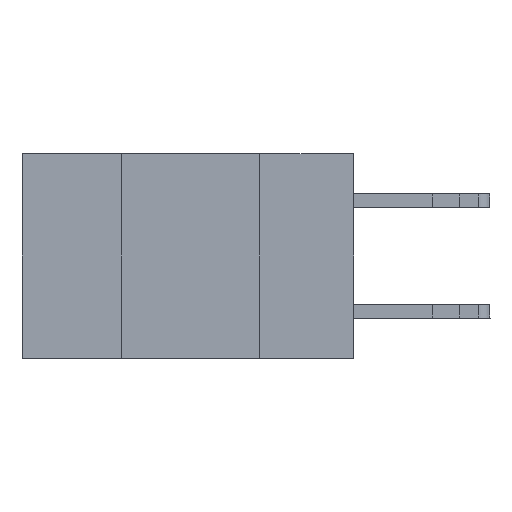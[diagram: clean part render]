
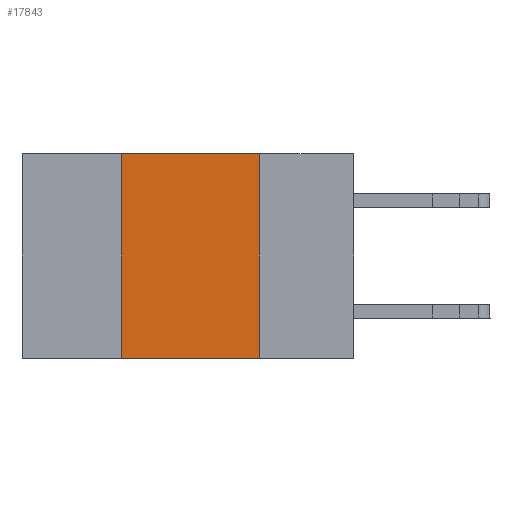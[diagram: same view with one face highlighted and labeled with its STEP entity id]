
A CAD part, left-side view. The second image highlights one B-rep face of the part: STEP entity #17843.
In plain terms, the highlighted planar face has unit normal (-1, 0, 0).
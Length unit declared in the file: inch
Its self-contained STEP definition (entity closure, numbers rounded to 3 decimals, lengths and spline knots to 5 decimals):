
#76 = CARTESIAN_POINT ( 'NONE',  ( 0., 0.6, 0. ) ) ;
#543 = ORIENTED_EDGE ( 'NONE', *, *, #3836, .F. ) ;
#1004 = LINE ( 'NONE', #16414, #1971 ) ;
#1146 = ORIENTED_EDGE ( 'NONE', *, *, #10322, .T. ) ;
#1477 = FACE_OUTER_BOUND ( 'NONE', #8916, .T. ) ;
#1574 = PLANE ( 'NONE',  #15258 ) ;
#1856 = CARTESIAN_POINT ( 'NONE',  ( 0., 0.42, 0. ) ) ;
#1971 = VECTOR ( 'NONE', #13468, 39.37008 ) ;
#2335 = CARTESIAN_POINT ( 'NONE',  ( 0., 0.42, -0.37 ) ) ;
#2457 = LINE ( 'NONE', #8667, #14725 ) ;
#3836 = EDGE_CURVE ( 'NONE', #6164, #16269, #12143, .T. ) ;
#4423 = DIRECTION ( 'NONE',  ( 1., 0., 0. ) ) ;
#5295 = CARTESIAN_POINT ( 'NONE',  ( 0., 0.17, -0.37 ) ) ;
#6164 = VERTEX_POINT ( 'NONE', #1856 ) ;
#7661 = LINE ( 'NONE', #13633, #12698 ) ;
#8169 = EDGE_CURVE ( 'NONE', #10997, #6164, #1004, .T. ) ;
#8365 = ORIENTED_EDGE ( 'NONE', *, *, #8169, .F. ) ;
#8667 = CARTESIAN_POINT ( 'NONE',  ( 0., 0.17, 0. ) ) ;
#8916 = EDGE_LOOP ( 'NONE', ( #16195, #543, #8365, #1146 ) ) ;
#10322 = EDGE_CURVE ( 'NONE', #10997, #15309, #7661, .T. ) ;
#10779 = DIRECTION ( 'NONE',  ( 0., 0., -1. ) ) ;
#10997 = VERTEX_POINT ( 'NONE', #2335 ) ;
#11593 = VECTOR ( 'NONE', #16829, 39.37008 ) ;
#12143 = LINE ( 'NONE', #18355, #11593 ) ;
#12698 = VECTOR ( 'NONE', #13937, 39.37008 ) ;
#12846 = CARTESIAN_POINT ( 'NONE',  ( 0., 0.17, 0. ) ) ;
#13468 = DIRECTION ( 'NONE',  ( 0., 0., 1. ) ) ;
#13633 = CARTESIAN_POINT ( 'NONE',  ( 0., 0.6, -0.37 ) ) ;
#13855 = DIRECTION ( 'NONE',  ( 0., 0., -1. ) ) ;
#13937 = DIRECTION ( 'NONE',  ( 0., -1., 0. ) ) ;
#14725 = VECTOR ( 'NONE', #10779, 39.37008 ) ;
#15258 = AXIS2_PLACEMENT_3D ( 'NONE', #76, #4423, #13855 ) ;
#15309 = VERTEX_POINT ( 'NONE', #5295 ) ;
#16195 = ORIENTED_EDGE ( 'NONE', *, *, #19655, .F. ) ;
#16269 = VERTEX_POINT ( 'NONE', #12846 ) ;
#16414 = CARTESIAN_POINT ( 'NONE',  ( 0., 0.42, 0. ) ) ;
#16829 = DIRECTION ( 'NONE',  ( 0., -1., 0. ) ) ;
#17843 = ADVANCED_FACE ( 'NONE', ( #1477 ), #1574, .F. ) ;
#18355 = CARTESIAN_POINT ( 'NONE',  ( 0., 0.6, 0. ) ) ;
#19655 = EDGE_CURVE ( 'NONE', #16269, #15309, #2457, .T. ) ;
